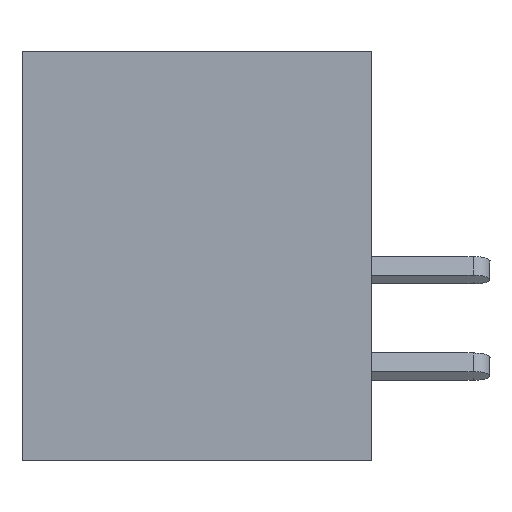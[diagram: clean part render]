
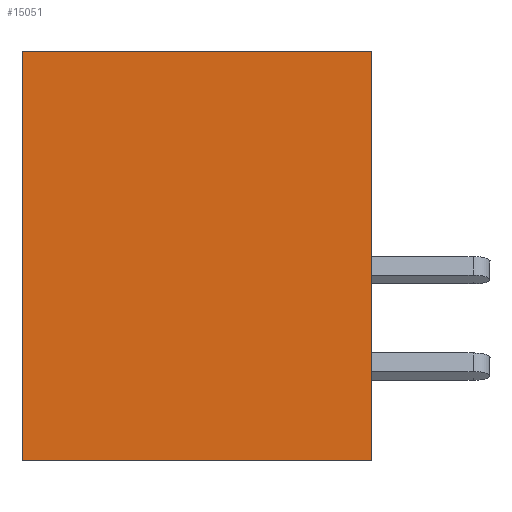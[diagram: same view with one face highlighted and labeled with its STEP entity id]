
A CAD part, left-side view. The second image highlights one B-rep face of the part: STEP entity #15051.
In plain terms, the highlighted planar face has unit normal (-1, 0, 0).
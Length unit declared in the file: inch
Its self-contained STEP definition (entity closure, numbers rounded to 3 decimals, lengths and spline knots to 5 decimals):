
#973 = VECTOR ( 'NONE', #8680, 39.37008 ) ;
#1324 = CARTESIAN_POINT ( 'NONE',  ( 0., 0.453, -0.531 ) ) ;
#1464 = CARTESIAN_POINT ( 'NONE',  ( 0., 0., -0.531 ) ) ;
#2326 = VECTOR ( 'NONE', #11836, 39.37008 ) ;
#3030 = EDGE_CURVE ( 'NONE', #5231, #14702, #8881, .T. ) ;
#3099 = EDGE_LOOP ( 'NONE', ( #4188, #5548, #9968, #14792 ) ) ;
#4188 = ORIENTED_EDGE ( 'NONE', *, *, #12779, .T. ) ;
#5231 = VERTEX_POINT ( 'NONE', #5915 ) ;
#5548 = ORIENTED_EDGE ( 'NONE', *, *, #3030, .F. ) ;
#5915 = CARTESIAN_POINT ( 'NONE',  ( 0., 0.453, 0. ) ) ;
#6756 = EDGE_CURVE ( 'NONE', #18723, #13507, #14740, .T. ) ;
#7059 = LINE ( 'NONE', #14360, #12914 ) ;
#7455 = CARTESIAN_POINT ( 'NONE',  ( 0., 0.453, 0. ) ) ;
#8471 = DIRECTION ( 'NONE',  ( 0., 0., 1. ) ) ;
#8680 = DIRECTION ( 'NONE',  ( 0., 0., 1. ) ) ;
#8836 = PLANE ( 'NONE',  #15761 ) ;
#8881 = LINE ( 'NONE', #11352, #12170 ) ;
#9046 = DIRECTION ( 'NONE',  ( 1., 0., 0. ) ) ;
#9968 = ORIENTED_EDGE ( 'NONE', *, *, #13209, .F. ) ;
#10347 = DIRECTION ( 'NONE',  ( 0., 0., -1. ) ) ;
#10433 = CARTESIAN_POINT ( 'NONE',  ( 0., 0.453, -0.531 ) ) ;
#11352 = CARTESIAN_POINT ( 'NONE',  ( 0., 0.453, 0. ) ) ;
#11836 = DIRECTION ( 'NONE',  ( 0., -1., 0. ) ) ;
#12170 = VECTOR ( 'NONE', #18556, 39.37008 ) ;
#12779 = EDGE_CURVE ( 'NONE', #13507, #14702, #18492, .T. ) ;
#12914 = VECTOR ( 'NONE', #8471, 39.37008 ) ;
#13209 = EDGE_CURVE ( 'NONE', #18723, #5231, #7059, .T. ) ;
#13507 = VERTEX_POINT ( 'NONE', #1464 ) ;
#14360 = CARTESIAN_POINT ( 'NONE',  ( 0., 0.453, 0. ) ) ;
#14702 = VERTEX_POINT ( 'NONE', #15322 ) ;
#14740 = LINE ( 'NONE', #1324, #2326 ) ;
#14792 = ORIENTED_EDGE ( 'NONE', *, *, #6756, .T. ) ;
#15051 = ADVANCED_FACE ( 'NONE', ( #16532 ), #8836, .F. ) ;
#15322 = CARTESIAN_POINT ( 'NONE',  ( 0., 0., 0. ) ) ;
#15761 = AXIS2_PLACEMENT_3D ( 'NONE', #7455, #9046, #10347 ) ;
#15795 = CARTESIAN_POINT ( 'NONE',  ( 0., 0., 0. ) ) ;
#16532 = FACE_OUTER_BOUND ( 'NONE', #3099, .T. ) ;
#18492 = LINE ( 'NONE', #15795, #973 ) ;
#18556 = DIRECTION ( 'NONE',  ( 0., -1., 0. ) ) ;
#18723 = VERTEX_POINT ( 'NONE', #10433 ) ;
